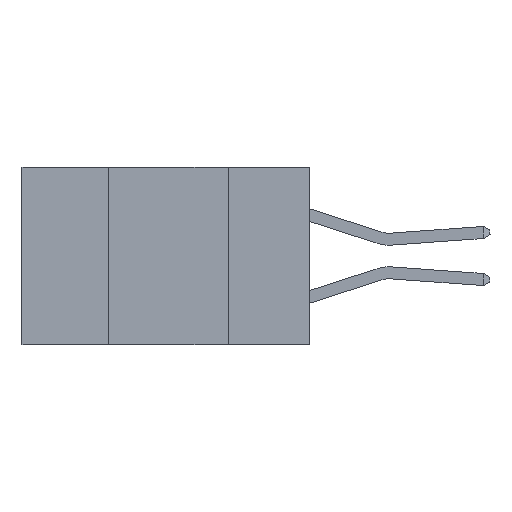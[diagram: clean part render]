
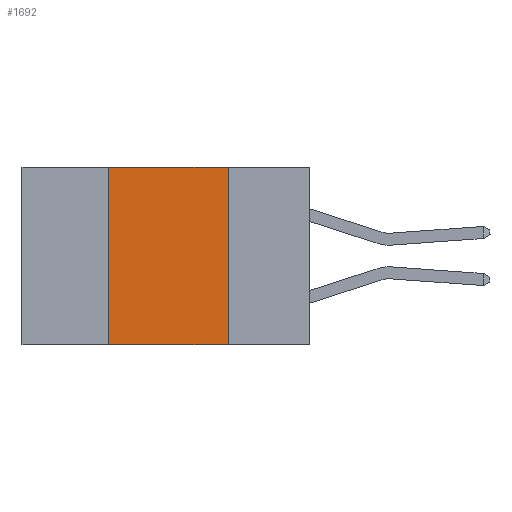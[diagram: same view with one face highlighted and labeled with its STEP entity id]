
A CAD part, left-side view. The second image highlights one B-rep face of the part: STEP entity #1692.
In plain terms, the highlighted planar face has unit normal (-1, 0, 0).
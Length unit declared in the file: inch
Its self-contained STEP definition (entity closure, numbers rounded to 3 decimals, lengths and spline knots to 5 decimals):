
#54 = PLANE ( 'NONE',  #13193 ) ;
#428 = ORIENTED_EDGE ( 'NONE', *, *, #6278, .F. ) ;
#1076 = VECTOR ( 'NONE', #6872, 39.37008 ) ;
#1267 = CARTESIAN_POINT ( 'NONE',  ( 0., 0.6, 0. ) ) ;
#1505 = VECTOR ( 'NONE', #8207, 39.37008 ) ;
#1581 = LINE ( 'NONE', #12918, #3566 ) ;
#1692 = ADVANCED_FACE ( 'NONE', ( #3878 ), #54, .F. ) ;
#1865 = CARTESIAN_POINT ( 'NONE',  ( 0., 0.17, 0. ) ) ;
#2240 = ORIENTED_EDGE ( 'NONE', *, *, #5402, .T. ) ;
#2387 = CARTESIAN_POINT ( 'NONE',  ( 0., 0.17, -0.37 ) ) ;
#3227 = VECTOR ( 'NONE', #4434, 39.37008 ) ;
#3566 = VECTOR ( 'NONE', #13007, 39.37008 ) ;
#3878 = FACE_OUTER_BOUND ( 'NONE', #5069, .T. ) ;
#4434 = DIRECTION ( 'NONE',  ( 0., 0., -1. ) ) ;
#5006 = ORIENTED_EDGE ( 'NONE', *, *, #11189, .F. ) ;
#5020 = DIRECTION ( 'NONE',  ( 0., 0., -1. ) ) ;
#5069 = EDGE_LOOP ( 'NONE', ( #12568, #5006, #428, #2240 ) ) ;
#5402 = EDGE_CURVE ( 'NONE', #13613, #14536, #6959, .T. ) ;
#6028 = DIRECTION ( 'NONE',  ( 1., 0., 0. ) ) ;
#6278 = EDGE_CURVE ( 'NONE', #13613, #14813, #1581, .T. ) ;
#6789 = CARTESIAN_POINT ( 'NONE',  ( 0., 0.17, -0.37 ) ) ;
#6872 = DIRECTION ( 'NONE',  ( 0., -1., 0. ) ) ;
#6959 = LINE ( 'NONE', #13805, #1076 ) ;
#8005 = VERTEX_POINT ( 'NONE', #1865 ) ;
#8207 = DIRECTION ( 'NONE',  ( 0., -1., 0. ) ) ;
#8915 = CARTESIAN_POINT ( 'NONE',  ( 0., 0.42, 0. ) ) ;
#9456 = CARTESIAN_POINT ( 'NONE',  ( 0., 0.6, 0. ) ) ;
#11189 = EDGE_CURVE ( 'NONE', #14813, #8005, #13004, .T. ) ;
#11284 = LINE ( 'NONE', #6789, #3227 ) ;
#12568 = ORIENTED_EDGE ( 'NONE', *, *, #14359, .F. ) ;
#12918 = CARTESIAN_POINT ( 'NONE',  ( 0., 0.42, -0.37 ) ) ;
#13004 = LINE ( 'NONE', #1267, #1505 ) ;
#13007 = DIRECTION ( 'NONE',  ( 0., 0., 1. ) ) ;
#13193 = AXIS2_PLACEMENT_3D ( 'NONE', #9456, #6028, #5020 ) ;
#13613 = VERTEX_POINT ( 'NONE', #15016 ) ;
#13805 = CARTESIAN_POINT ( 'NONE',  ( 0., 0.6, -0.37 ) ) ;
#14359 = EDGE_CURVE ( 'NONE', #8005, #14536, #11284, .T. ) ;
#14536 = VERTEX_POINT ( 'NONE', #2387 ) ;
#14813 = VERTEX_POINT ( 'NONE', #8915 ) ;
#15016 = CARTESIAN_POINT ( 'NONE',  ( 0., 0.42, -0.37 ) ) ;
